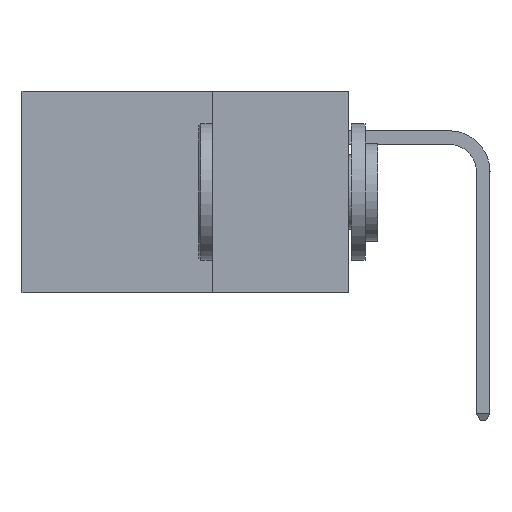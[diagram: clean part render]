
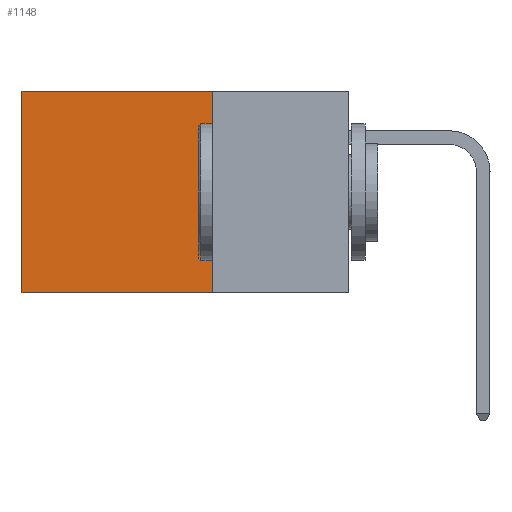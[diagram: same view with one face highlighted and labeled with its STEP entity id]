
A CAD part, left-side view. The second image highlights one B-rep face of the part: STEP entity #1148.
In plain terms, the highlighted planar face has unit normal (-1, 0, 0).
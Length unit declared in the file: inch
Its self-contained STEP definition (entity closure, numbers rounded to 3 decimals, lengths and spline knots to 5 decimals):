
#1148 = ADVANCED_FACE ( 'NONE', ( #14202 ), #21878, .F. ) ;
#1571 = CARTESIAN_POINT ( 'NONE',  ( 0.2875, 0.6, 0. ) ) ;
#2486 = DIRECTION ( 'NONE',  ( 1., 0., 0. ) ) ;
#2982 = CARTESIAN_POINT ( 'NONE',  ( 0.2875, 0.6, -0.37 ) ) ;
#3044 = ORIENTED_EDGE ( 'NONE', *, *, #19686, .F. ) ;
#5497 = DIRECTION ( 'NONE',  ( 0., 0., -1. ) ) ;
#8692 = CARTESIAN_POINT ( 'NONE',  ( 0.2875, 0.6, 0. ) ) ;
#12917 = VECTOR ( 'NONE', #17920, 39.37008 ) ;
#14136 = DIRECTION ( 'NONE',  ( 0., 1., 0. ) ) ;
#14202 = FACE_OUTER_BOUND ( 'NONE', #43216, .T. ) ;
#14543 = CARTESIAN_POINT ( 'NONE',  ( 0.2875, 0.25, -0.37 ) ) ;
#17602 = VERTEX_POINT ( 'NONE', #8692 ) ;
#17920 = DIRECTION ( 'NONE',  ( 0., 0., -1. ) ) ;
#18165 = LINE ( 'NONE', #33431, #28458 ) ;
#18607 = VERTEX_POINT ( 'NONE', #2982 ) ;
#19686 = EDGE_CURVE ( 'NONE', #37833, #18607, #18165, .T. ) ;
#20906 = EDGE_CURVE ( 'NONE', #36656, #17602, #40790, .T. ) ;
#21878 = PLANE ( 'NONE',  #41252 ) ;
#23204 = LINE ( 'NONE', #44976, #12917 ) ;
#28060 = LINE ( 'NONE', #1571, #47435 ) ;
#28458 = VECTOR ( 'NONE', #14136, 39.37008 ) ;
#28813 = ORIENTED_EDGE ( 'NONE', *, *, #20906, .T. ) ;
#29656 = DIRECTION ( 'NONE',  ( 0., 0., -1. ) ) ;
#33431 = CARTESIAN_POINT ( 'NONE',  ( 0.2875, 0.25, -0.37 ) ) ;
#35051 = ORIENTED_EDGE ( 'NONE', *, *, #42509, .T. ) ;
#36656 = VERTEX_POINT ( 'NONE', #50010 ) ;
#37833 = VERTEX_POINT ( 'NONE', #14543 ) ;
#38203 = DIRECTION ( 'NONE',  ( 0., 1., 0. ) ) ;
#39557 = VECTOR ( 'NONE', #38203, 39.37008 ) ;
#40790 = LINE ( 'NONE', #42079, #39557 ) ;
#41252 = AXIS2_PLACEMENT_3D ( 'NONE', #48942, #2486, #29656 ) ;
#42079 = CARTESIAN_POINT ( 'NONE',  ( 0.2875, 0.25, 0. ) ) ;
#42509 = EDGE_CURVE ( 'NONE', #17602, #18607, #28060, .T. ) ;
#43216 = EDGE_LOOP ( 'NONE', ( #35051, #3044, #46062, #28813 ) ) ;
#44976 = CARTESIAN_POINT ( 'NONE',  ( 0.2875, 0.25, 0. ) ) ;
#46062 = ORIENTED_EDGE ( 'NONE', *, *, #48031, .F. ) ;
#47435 = VECTOR ( 'NONE', #5497, 39.37008 ) ;
#48031 = EDGE_CURVE ( 'NONE', #36656, #37833, #23204, .T. ) ;
#48942 = CARTESIAN_POINT ( 'NONE',  ( 0.2875, 0.25, 0. ) ) ;
#50010 = CARTESIAN_POINT ( 'NONE',  ( 0.2875, 0.25, 0. ) ) ;
